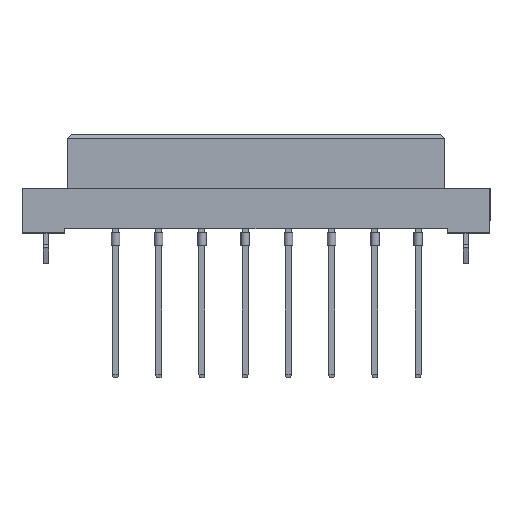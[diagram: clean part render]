
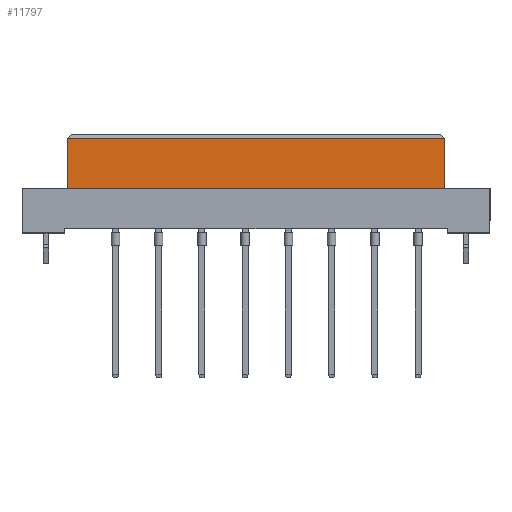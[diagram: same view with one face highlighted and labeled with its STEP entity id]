
A CAD part, top view. The second image highlights one B-rep face of the part: STEP entity #11797.
In plain terms, the highlighted planar face has unit normal (0, 0, 1).
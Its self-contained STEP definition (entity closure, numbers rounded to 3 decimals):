
#139 = EDGE_CURVE ( 'NONE', #6501, #21321, #7799, .T. ) ;
#952 = CARTESIAN_POINT ( 'NONE',  ( -22.2, -0.5, 4.25 ) ) ;
#1307 = VECTOR ( 'NONE', #19204, 1000. ) ;
#2394 = CARTESIAN_POINT ( 'NONE',  ( 22.2, -6.4, 4.25 ) ) ;
#2982 = DIRECTION ( 'NONE',  ( 0., 1., 0. ) ) ;
#3680 = EDGE_CURVE ( 'NONE', #14639, #21419, #16099, .T. ) ;
#4109 = VECTOR ( 'NONE', #2982, 1000. ) ;
#4613 = LINE ( 'NONE', #17868, #4109 ) ;
#5213 = ORIENTED_EDGE ( 'NONE', *, *, #3680, .T. ) ;
#5777 = ORIENTED_EDGE ( 'NONE', *, *, #139, .T. ) ;
#6069 = VECTOR ( 'NONE', #6701, 1000. ) ;
#6501 = VERTEX_POINT ( 'NONE', #13906 ) ;
#6701 = DIRECTION ( 'NONE',  ( 0., 1., 0. ) ) ;
#6741 = AXIS2_PLACEMENT_3D ( 'NONE', #19209, #12487, #15844 ) ;
#7209 = VECTOR ( 'NONE', #20872, 1000. ) ;
#7799 = LINE ( 'NONE', #18979, #1307 ) ;
#7976 = ORIENTED_EDGE ( 'NONE', *, *, #10703, .T. ) ;
#9952 = CARTESIAN_POINT ( 'NONE',  ( -22.2, -6.4, 4.25 ) ) ;
#10061 = LINE ( 'NONE', #21457, #6069 ) ;
#10703 = EDGE_CURVE ( 'NONE', #21419, #6501, #4613, .T. ) ;
#10952 = PLANE ( 'NONE',  #6741 ) ;
#11068 = CARTESIAN_POINT ( 'NONE',  ( 22.2, -6.4, 4.25 ) ) ;
#11797 = ADVANCED_FACE ( 'NONE', ( #15953 ), #10952, .T. ) ;
#11975 = EDGE_CURVE ( 'NONE', #14639, #21321, #10061, .T. ) ;
#12487 = DIRECTION ( 'NONE',  ( 0., 0., 1. ) ) ;
#13906 = CARTESIAN_POINT ( 'NONE',  ( 22.2, -0.5, 4.25 ) ) ;
#14054 = EDGE_LOOP ( 'NONE', ( #7976, #5777, #20386, #5213 ) ) ;
#14639 = VERTEX_POINT ( 'NONE', #9952 ) ;
#15844 = DIRECTION ( 'NONE',  ( 1., 0., 0. ) ) ;
#15953 = FACE_OUTER_BOUND ( 'NONE', #14054, .T. ) ;
#16099 = LINE ( 'NONE', #2394, #7209 ) ;
#17868 = CARTESIAN_POINT ( 'NONE',  ( 22.2, -6.4, 4.25 ) ) ;
#18979 = CARTESIAN_POINT ( 'NONE',  ( -22.2, -0.5, 4.25 ) ) ;
#19204 = DIRECTION ( 'NONE',  ( -1., 0., 0. ) ) ;
#19209 = CARTESIAN_POINT ( 'NONE',  ( 22.2, -6.4, 4.25 ) ) ;
#20386 = ORIENTED_EDGE ( 'NONE', *, *, #11975, .F. ) ;
#20872 = DIRECTION ( 'NONE',  ( 1., 0., 0. ) ) ;
#21321 = VERTEX_POINT ( 'NONE', #952 ) ;
#21419 = VERTEX_POINT ( 'NONE', #11068 ) ;
#21457 = CARTESIAN_POINT ( 'NONE',  ( -22.2, -6.4, 4.25 ) ) ;
